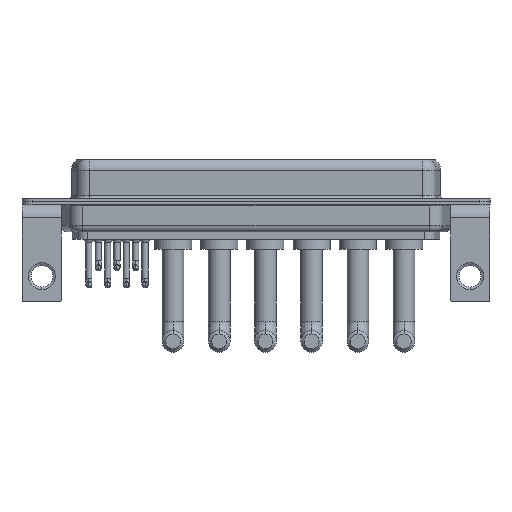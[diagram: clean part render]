
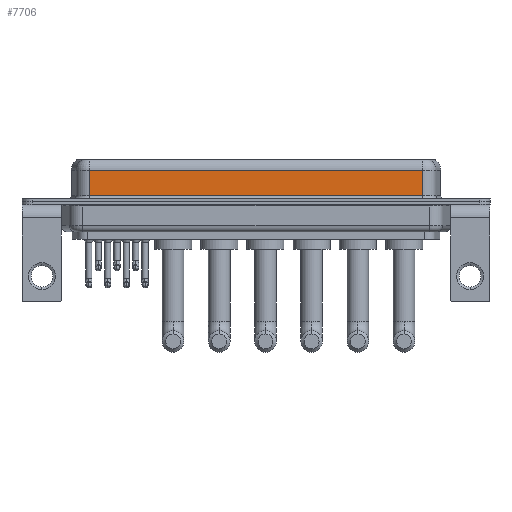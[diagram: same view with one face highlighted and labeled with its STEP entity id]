
A CAD part, front view. The second image highlights one B-rep face of the part: STEP entity #7706.
In plain terms, the highlighted planar face has unit normal (0, -1, 0).
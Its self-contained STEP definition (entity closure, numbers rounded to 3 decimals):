
#524 = DIRECTION ( 'NONE',  ( -1., 0., 0. ) ) ;
#1216 = LINE ( 'NONE', #2495, #14926 ) ;
#1410 = EDGE_CURVE ( 'NONE', #12478, #3783, #1216, .T. ) ;
#1900 = CARTESIAN_POINT ( 'NONE',  ( 56.462, -3.95, 4.65 ) ) ;
#2495 = CARTESIAN_POINT ( 'NONE',  ( 56.462, -3.95, 6.4 ) ) ;
#2617 = ORIENTED_EDGE ( 'NONE', *, *, #5732, .T. ) ;
#3364 = VECTOR ( 'NONE', #524, 1000. ) ;
#3783 = VERTEX_POINT ( 'NONE', #17103 ) ;
#3997 = DIRECTION ( 'NONE',  ( 0., 0., 1. ) ) ;
#4068 = VERTEX_POINT ( 'NONE', #10046 ) ;
#4446 = EDGE_CURVE ( 'NONE', #4849, #3783, #19030, .T. ) ;
#4849 = VERTEX_POINT ( 'NONE', #16192 ) ;
#5508 = DIRECTION ( 'NONE',  ( 0., 0., -1. ) ) ;
#5732 = EDGE_CURVE ( 'NONE', #4068, #4849, #17226, .T. ) ;
#5739 = AXIS2_PLACEMENT_3D ( 'NONE', #16223, #8850, #3997 ) ;
#6437 = ORIENTED_EDGE ( 'NONE', *, *, #13420, .T. ) ;
#7113 = ORIENTED_EDGE ( 'NONE', *, *, #1410, .F. ) ;
#7706 = ADVANCED_FACE ( 'NONE', ( #17589 ), #19116, .F. ) ;
#8497 = CARTESIAN_POINT ( 'NONE',  ( 7.038, -3.95, 6.4 ) ) ;
#8850 = DIRECTION ( 'NONE',  ( 0., 1., 0. ) ) ;
#8859 = DIRECTION ( 'NONE',  ( 1., 0., 0. ) ) ;
#9866 = VECTOR ( 'NONE', #12540, 1000. ) ;
#10046 = CARTESIAN_POINT ( 'NONE',  ( 7.038, -3.95, 4.65 ) ) ;
#10542 = EDGE_LOOP ( 'NONE', ( #7113, #6437, #2617, #15557 ) ) ;
#12478 = VERTEX_POINT ( 'NONE', #17859 ) ;
#12540 = DIRECTION ( 'NONE',  ( 0., 0., -1. ) ) ;
#13292 = CARTESIAN_POINT ( 'NONE',  ( 56.462, -3.95, 0.9 ) ) ;
#13420 = EDGE_CURVE ( 'NONE', #12478, #4068, #13833, .T. ) ;
#13833 = LINE ( 'NONE', #1900, #3364 ) ;
#14926 = VECTOR ( 'NONE', #5508, 1000. ) ;
#15510 = VECTOR ( 'NONE', #8859, 1000. ) ;
#15557 = ORIENTED_EDGE ( 'NONE', *, *, #4446, .T. ) ;
#16192 = CARTESIAN_POINT ( 'NONE',  ( 7.038, -3.95, 0.9 ) ) ;
#16223 = CARTESIAN_POINT ( 'NONE',  ( 56.462, -3.95, 6.4 ) ) ;
#17103 = CARTESIAN_POINT ( 'NONE',  ( 56.462, -3.95, 0.9 ) ) ;
#17226 = LINE ( 'NONE', #8497, #9866 ) ;
#17589 = FACE_OUTER_BOUND ( 'NONE', #10542, .T. ) ;
#17859 = CARTESIAN_POINT ( 'NONE',  ( 56.462, -3.95, 4.65 ) ) ;
#19030 = LINE ( 'NONE', #13292, #15510 ) ;
#19116 = PLANE ( 'NONE',  #5739 ) ;
